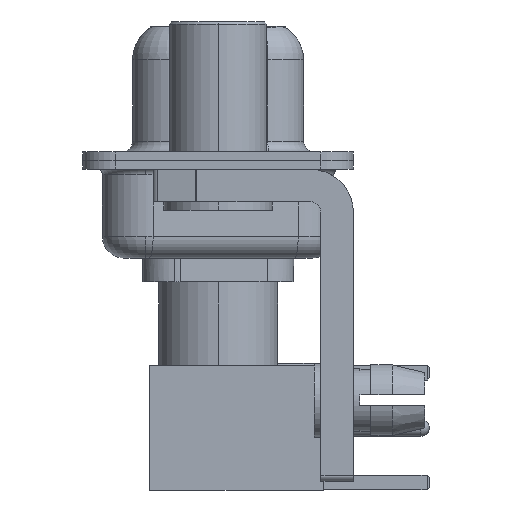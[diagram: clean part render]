
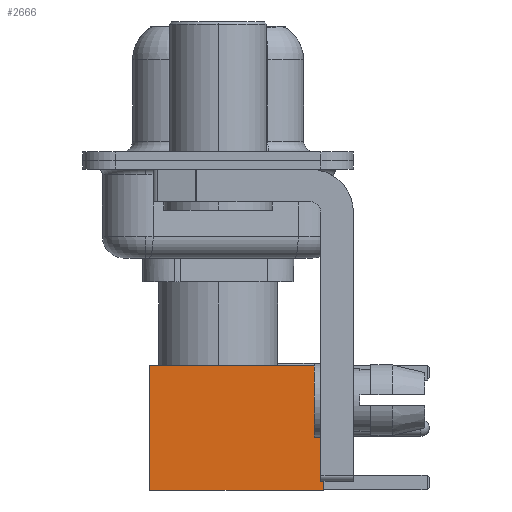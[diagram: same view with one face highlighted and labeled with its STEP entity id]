
A CAD part, left-side view. The second image highlights one B-rep face of the part: STEP entity #2666.
In plain terms, the highlighted face is planar.
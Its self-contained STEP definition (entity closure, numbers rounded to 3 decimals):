
#1003 = CARTESIAN_POINT ( 'NONE',  ( 2.875, 2.875, 8. ) ) ;
#1451 = LINE ( 'NONE', #7626, #26649 ) ;
#1676 = DIRECTION ( 'NONE',  ( 0., 1., 0. ) ) ;
#1784 = EDGE_CURVE ( 'NONE', #9255, #21298, #12145, .T. ) ;
#2666 = ADVANCED_FACE ( 'NONE', ( #22914 ), #3642, .T. ) ;
#3642 = PLANE ( 'NONE',  #23345 ) ;
#4784 = DIRECTION ( 'NONE',  ( -1., 0., 0. ) ) ;
#4806 = CARTESIAN_POINT ( 'NONE',  ( -2.875, 2.875, 0. ) ) ;
#6725 = ORIENTED_EDGE ( 'NONE', *, *, #20220, .F. ) ;
#7178 = LINE ( 'NONE', #4806, #14701 ) ;
#7626 = CARTESIAN_POINT ( 'NONE',  ( 0., 2.875, 0. ) ) ;
#8050 = DIRECTION ( 'NONE',  ( 0., 0., -1. ) ) ;
#8672 = ORIENTED_EDGE ( 'NONE', *, *, #15001, .F. ) ;
#9255 = VERTEX_POINT ( 'NONE', #1003 ) ;
#11783 = ORIENTED_EDGE ( 'NONE', *, *, #22633, .T. ) ;
#12145 = LINE ( 'NONE', #27350, #22456 ) ;
#12212 = CARTESIAN_POINT ( 'NONE',  ( 2.875, 2.875, 0. ) ) ;
#13172 = CARTESIAN_POINT ( 'NONE',  ( -2.875, 2.875, 8. ) ) ;
#14701 = VECTOR ( 'NONE', #22237, 1000. ) ;
#15001 = EDGE_CURVE ( 'NONE', #21605, #27399, #7178, .T. ) ;
#16268 = ORIENTED_EDGE ( 'NONE', *, *, #1784, .T. ) ;
#16616 = CARTESIAN_POINT ( 'NONE',  ( -2.875, 2.875, 0. ) ) ;
#17117 = VECTOR ( 'NONE', #4784, 1000. ) ;
#17321 = LINE ( 'NONE', #24047, #17117 ) ;
#18626 = DIRECTION ( 'NONE',  ( -1., 0., 0. ) ) ;
#19252 = CARTESIAN_POINT ( 'NONE',  ( 2.875, 2.875, 0. ) ) ;
#20220 = EDGE_CURVE ( 'NONE', #9255, #21605, #17321, .T. ) ;
#20805 = EDGE_LOOP ( 'NONE', ( #16268, #11783, #8672, #6725 ) ) ;
#21298 = VERTEX_POINT ( 'NONE', #19252 ) ;
#21605 = VERTEX_POINT ( 'NONE', #13172 ) ;
#22237 = DIRECTION ( 'NONE',  ( 0., 0., -1. ) ) ;
#22456 = VECTOR ( 'NONE', #8050, 1000. ) ;
#22633 = EDGE_CURVE ( 'NONE', #21298, #27399, #1451, .T. ) ;
#22914 = FACE_OUTER_BOUND ( 'NONE', #20805, .T. ) ;
#23345 = AXIS2_PLACEMENT_3D ( 'NONE', #12212, #1676, #27418 ) ;
#24047 = CARTESIAN_POINT ( 'NONE',  ( 0., 2.875, 8. ) ) ;
#26649 = VECTOR ( 'NONE', #18626, 1000. ) ;
#27350 = CARTESIAN_POINT ( 'NONE',  ( 2.875, 2.875, 0. ) ) ;
#27399 = VERTEX_POINT ( 'NONE', #16616 ) ;
#27418 = DIRECTION ( 'NONE',  ( 0., 0., 1. ) ) ;
